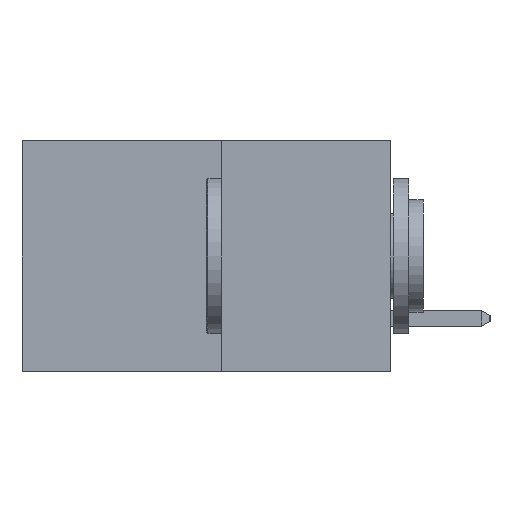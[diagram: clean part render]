
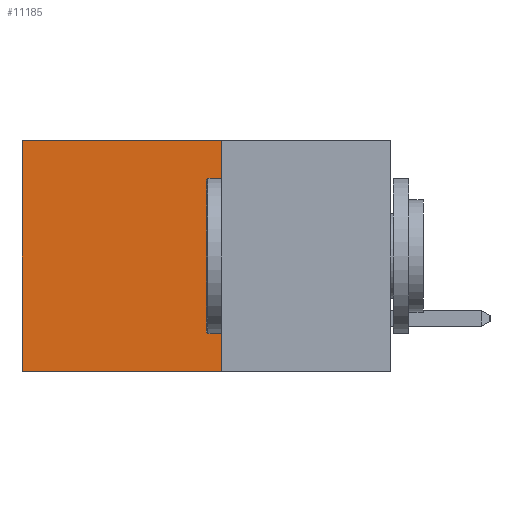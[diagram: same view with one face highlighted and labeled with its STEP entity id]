
A CAD part, left-side view. The second image highlights one B-rep face of the part: STEP entity #11185.
In plain terms, the highlighted planar face has unit normal (-1, 0, 0).
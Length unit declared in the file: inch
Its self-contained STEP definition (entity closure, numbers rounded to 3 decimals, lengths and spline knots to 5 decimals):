
#346 = VERTEX_POINT ( 'NONE', #11744 ) ;
#721 = DIRECTION ( 'NONE',  ( 0., 0., -1. ) ) ;
#967 = CARTESIAN_POINT ( 'NONE',  ( 0.277, 0.59, -0.37 ) ) ;
#1155 = EDGE_CURVE ( 'NONE', #15606, #16391, #9287, .T. ) ;
#2089 = VECTOR ( 'NONE', #7368, 39.37008 ) ;
#3515 = DIRECTION ( 'NONE',  ( 0., 1., 0. ) ) ;
#3786 = EDGE_LOOP ( 'NONE', ( #14163, #4208, #9032, #4116 ) ) ;
#3991 = LINE ( 'NONE', #11592, #17473 ) ;
#4064 = VECTOR ( 'NONE', #721, 39.37008 ) ;
#4112 = PLANE ( 'NONE',  #17125 ) ;
#4116 = ORIENTED_EDGE ( 'NONE', *, *, #1155, .T. ) ;
#4208 = ORIENTED_EDGE ( 'NONE', *, *, #13369, .F. ) ;
#4954 = EDGE_CURVE ( 'NONE', #16391, #11650, #7676, .T. ) ;
#5488 = DIRECTION ( 'NONE',  ( 0., 0., -1. ) ) ;
#5725 = VECTOR ( 'NONE', #10851, 39.37008 ) ;
#5992 = CARTESIAN_POINT ( 'NONE',  ( 0.277, 0.27, -0.37 ) ) ;
#7368 = DIRECTION ( 'NONE',  ( 0., 0., -1. ) ) ;
#7450 = FACE_OUTER_BOUND ( 'NONE', #3786, .T. ) ;
#7676 = LINE ( 'NONE', #967, #4064 ) ;
#9032 = ORIENTED_EDGE ( 'NONE', *, *, #11922, .F. ) ;
#9287 = LINE ( 'NONE', #14181, #5725 ) ;
#9473 = CARTESIAN_POINT ( 'NONE',  ( 0.277, 0.27, -0.37 ) ) ;
#10346 = CARTESIAN_POINT ( 'NONE',  ( 0.277, 0.59, -0.37 ) ) ;
#10851 = DIRECTION ( 'NONE',  ( 0., 1., 0. ) ) ;
#11185 = ADVANCED_FACE ( 'NONE', ( #7450 ), #4112, .F. ) ;
#11592 = CARTESIAN_POINT ( 'NONE',  ( 0.277, 0.27, -0.37 ) ) ;
#11650 = VERTEX_POINT ( 'NONE', #10346 ) ;
#11744 = CARTESIAN_POINT ( 'NONE',  ( 0.277, 0.27, -0.37 ) ) ;
#11922 = EDGE_CURVE ( 'NONE', #15606, #346, #12888, .T. ) ;
#12888 = LINE ( 'NONE', #5992, #2089 ) ;
#13369 = EDGE_CURVE ( 'NONE', #346, #11650, #3991, .T. ) ;
#13543 = DIRECTION ( 'NONE',  ( 1., 0., 0. ) ) ;
#14163 = ORIENTED_EDGE ( 'NONE', *, *, #4954, .T. ) ;
#14181 = CARTESIAN_POINT ( 'NONE',  ( 0.277, 0.27, 0. ) ) ;
#14830 = CARTESIAN_POINT ( 'NONE',  ( 0.277, 0.59, 0. ) ) ;
#15606 = VERTEX_POINT ( 'NONE', #15982 ) ;
#15982 = CARTESIAN_POINT ( 'NONE',  ( 0.277, 0.27, 0. ) ) ;
#16391 = VERTEX_POINT ( 'NONE', #14830 ) ;
#17125 = AXIS2_PLACEMENT_3D ( 'NONE', #9473, #13543, #5488 ) ;
#17473 = VECTOR ( 'NONE', #3515, 39.37008 ) ;
